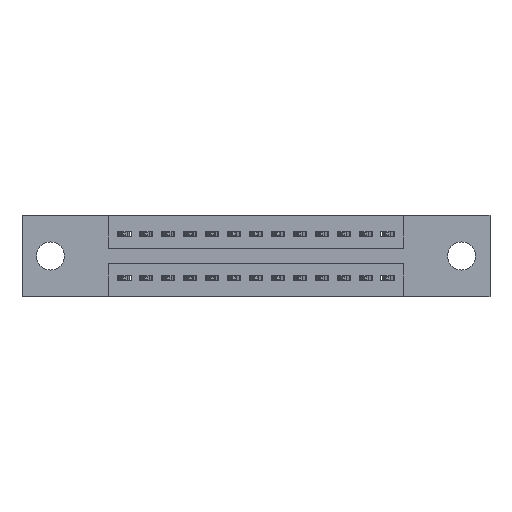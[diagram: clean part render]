
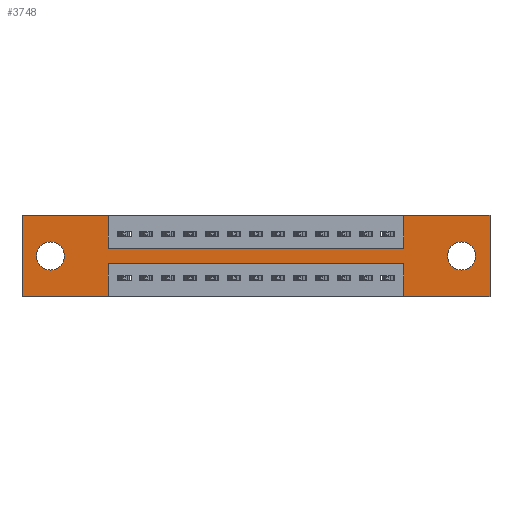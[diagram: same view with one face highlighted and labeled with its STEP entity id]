
A CAD part, front view. The second image highlights one B-rep face of the part: STEP entity #3748.
In plain terms, the highlighted planar face has unit normal (0, -1, 0).
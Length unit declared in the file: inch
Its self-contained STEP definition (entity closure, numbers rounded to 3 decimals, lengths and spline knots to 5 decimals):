
#61 = EDGE_CURVE ( 'NONE', #3490, #3423, #10278, .T. ) ;
#77 = VERTEX_POINT ( 'NONE', #11691 ) ;
#317 = DIRECTION ( 'NONE',  ( 0., 0., -1. ) ) ;
#356 = CARTESIAN_POINT ( 'NONE',  ( 0., 0., -0.37 ) ) ;
#383 = ORIENTED_EDGE ( 'NONE', *, *, #7710, .F. ) ;
#387 = VERTEX_POINT ( 'NONE', #8515 ) ;
#494 = DIRECTION ( 'NONE',  ( 0., 0., 1. ) ) ;
#524 = CARTESIAN_POINT ( 'NONE',  ( 0.13, 0., -0.185 ) ) ;
#543 = LINE ( 'NONE', #12159, #6457 ) ;
#552 = CARTESIAN_POINT ( 'NONE',  ( 1.7425, 0., 0. ) ) ;
#1044 = EDGE_CURVE ( 'NONE', #3004, #1251, #7736, .T. ) ;
#1169 = VERTEX_POINT ( 'NONE', #552 ) ;
#1219 = ORIENTED_EDGE ( 'NONE', *, *, #2390, .F. ) ;
#1251 = VERTEX_POINT ( 'NONE', #9426 ) ;
#1359 = DIRECTION ( 'NONE',  ( 1., 0., 0. ) ) ;
#1481 = CARTESIAN_POINT ( 'NONE',  ( 0., 0., 0. ) ) ;
#1528 = DIRECTION ( 'NONE',  ( 0., 0., 1. ) ) ;
#1544 = CIRCLE ( 'NONE', #6856, 0.064 ) ;
#1558 = DIRECTION ( 'NONE',  ( -1., 0., 0. ) ) ;
#1651 = EDGE_CURVE ( 'NONE', #13113, #387, #5462, .T. ) ;
#1752 = FACE_OUTER_BOUND ( 'NONE', #13735, .T. ) ;
#1858 = DIRECTION ( 'NONE',  ( 0., 0., 1. ) ) ;
#1883 = CARTESIAN_POINT ( 'NONE',  ( 2.135, 0., -0.37 ) ) ;
#1979 = VECTOR ( 'NONE', #1359, 39.37008 ) ;
#2236 = CARTESIAN_POINT ( 'NONE',  ( 2.135, 0., 0. ) ) ;
#2390 = EDGE_CURVE ( 'NONE', #8457, #4917, #5078, .T. ) ;
#2726 = CARTESIAN_POINT ( 'NONE',  ( 0.3925, 0., -0.15 ) ) ;
#2731 = CARTESIAN_POINT ( 'NONE',  ( 1.7425, 0., 0. ) ) ;
#2980 = LINE ( 'NONE', #12984, #13831 ) ;
#2991 = ORIENTED_EDGE ( 'NONE', *, *, #12994, .T. ) ;
#3004 = VERTEX_POINT ( 'NONE', #14059 ) ;
#3158 = AXIS2_PLACEMENT_3D ( 'NONE', #10783, #7246, #7576 ) ;
#3216 = CARTESIAN_POINT ( 'NONE',  ( 0.13, 0., -0.249 ) ) ;
#3333 = ORIENTED_EDGE ( 'NONE', *, *, #11763, .F. ) ;
#3414 = DIRECTION ( 'NONE',  ( 0., 0., -1. ) ) ;
#3423 = VERTEX_POINT ( 'NONE', #8905 ) ;
#3490 = VERTEX_POINT ( 'NONE', #7966 ) ;
#3528 = EDGE_CURVE ( 'NONE', #3423, #3490, #1544, .T. ) ;
#3617 = VECTOR ( 'NONE', #1558, 39.37008 ) ;
#3696 = ORIENTED_EDGE ( 'NONE', *, *, #7559, .F. ) ;
#3748 = ADVANCED_FACE ( 'NONE', ( #7465, #5228, #1752 ), #5443, .T. ) ;
#3947 = LINE ( 'NONE', #6393, #6555 ) ;
#4068 = ORIENTED_EDGE ( 'NONE', *, *, #10423, .F. ) ;
#4096 = VECTOR ( 'NONE', #12613, 39.37008 ) ;
#4218 = VECTOR ( 'NONE', #13090, 39.37008 ) ;
#4289 = EDGE_CURVE ( 'NONE', #1251, #9823, #12178, .T. ) ;
#4331 = AXIS2_PLACEMENT_3D ( 'NONE', #5634, #5425, #5401 ) ;
#4567 = LINE ( 'NONE', #12171, #4218 ) ;
#4735 = CARTESIAN_POINT ( 'NONE',  ( 0.3925, 0., -0.22 ) ) ;
#4736 = DIRECTION ( 'NONE',  ( 0., 0., 1. ) ) ;
#4754 = DIRECTION ( 'NONE',  ( 0., 1., 0. ) ) ;
#4758 = CARTESIAN_POINT ( 'NONE',  ( 0.13, 0., -0.185 ) ) ;
#4917 = VERTEX_POINT ( 'NONE', #12175 ) ;
#5078 = LINE ( 'NONE', #1481, #1979 ) ;
#5228 = FACE_BOUND ( 'NONE', #8115, .T. ) ;
#5284 = CARTESIAN_POINT ( 'NONE',  ( 0., 0., 0. ) ) ;
#5348 = EDGE_CURVE ( 'NONE', #4917, #5632, #13626, .T. ) ;
#5401 = DIRECTION ( 'NONE',  ( 0., 0., -1. ) ) ;
#5425 = DIRECTION ( 'NONE',  ( 0., -1., 0. ) ) ;
#5443 = PLANE ( 'NONE',  #4331 ) ;
#5462 = CIRCLE ( 'NONE', #7497, 0.064 ) ;
#5632 = VERTEX_POINT ( 'NONE', #2726 ) ;
#5634 = CARTESIAN_POINT ( 'NONE',  ( 0., 0., -0.37 ) ) ;
#5644 = ORIENTED_EDGE ( 'NONE', *, *, #3528, .T. ) ;
#5851 = LINE ( 'NONE', #2731, #11211 ) ;
#5983 = ORIENTED_EDGE ( 'NONE', *, *, #1651, .T. ) ;
#6333 = ORIENTED_EDGE ( 'NONE', *, *, #11100, .F. ) ;
#6393 = CARTESIAN_POINT ( 'NONE',  ( 0., 0., 0. ) ) ;
#6457 = VECTOR ( 'NONE', #13072, 39.37008 ) ;
#6555 = VECTOR ( 'NONE', #494, 39.37008 ) ;
#6856 = AXIS2_PLACEMENT_3D ( 'NONE', #7679, #7663, #7643 ) ;
#6888 = CARTESIAN_POINT ( 'NONE',  ( 0.3925, 0., -0.37 ) ) ;
#6919 = DIRECTION ( 'NONE',  ( -1., 0., 0. ) ) ;
#6994 = EDGE_CURVE ( 'NONE', #9823, #8457, #3947, .T. ) ;
#7037 = VERTEX_POINT ( 'NONE', #1883 ) ;
#7058 = CARTESIAN_POINT ( 'NONE',  ( 2.135, 0., 0. ) ) ;
#7246 = DIRECTION ( 'NONE',  ( 0., 1., 0. ) ) ;
#7379 = VECTOR ( 'NONE', #317, 39.37008 ) ;
#7380 = ORIENTED_EDGE ( 'NONE', *, *, #6994, .F. ) ;
#7465 = FACE_BOUND ( 'NONE', #13155, .T. ) ;
#7497 = AXIS2_PLACEMENT_3D ( 'NONE', #4758, #4754, #4736 ) ;
#7559 = EDGE_CURVE ( 'NONE', #8117, #1169, #5851, .T. ) ;
#7576 = DIRECTION ( 'NONE',  ( 0., 0., -1. ) ) ;
#7643 = DIRECTION ( 'NONE',  ( 0., 0., -1. ) ) ;
#7663 = DIRECTION ( 'NONE',  ( 0., 1., 0. ) ) ;
#7679 = CARTESIAN_POINT ( 'NONE',  ( 2.005, 0., -0.185 ) ) ;
#7685 = LINE ( 'NONE', #2236, #12773 ) ;
#7710 = EDGE_CURVE ( 'NONE', #1169, #11822, #7771, .T. ) ;
#7736 = LINE ( 'NONE', #6888, #7379 ) ;
#7771 = LINE ( 'NONE', #5284, #4096 ) ;
#7966 = CARTESIAN_POINT ( 'NONE',  ( 2.005, 0., -0.249 ) ) ;
#8115 = EDGE_LOOP ( 'NONE', ( #2991, #5983 ) ) ;
#8117 = VERTEX_POINT ( 'NONE', #9492 ) ;
#8205 = CIRCLE ( 'NONE', #9465, 0.064 ) ;
#8457 = VERTEX_POINT ( 'NONE', #11938 ) ;
#8515 = CARTESIAN_POINT ( 'NONE',  ( 0.13, 0., -0.121 ) ) ;
#8614 = ORIENTED_EDGE ( 'NONE', *, *, #61, .T. ) ;
#8682 = DIRECTION ( 'NONE',  ( 0., 1., 0. ) ) ;
#8905 = CARTESIAN_POINT ( 'NONE',  ( 2.005, 0., -0.121 ) ) ;
#8969 = ORIENTED_EDGE ( 'NONE', *, *, #1044, .F. ) ;
#9307 = ORIENTED_EDGE ( 'NONE', *, *, #9521, .F. ) ;
#9426 = CARTESIAN_POINT ( 'NONE',  ( 0.3925, 0., -0.37 ) ) ;
#9465 = AXIS2_PLACEMENT_3D ( 'NONE', #524, #8682, #1858 ) ;
#9492 = CARTESIAN_POINT ( 'NONE',  ( 1.7425, 0., -0.15 ) ) ;
#9521 = EDGE_CURVE ( 'NONE', #7037, #77, #4567, .T. ) ;
#9823 = VERTEX_POINT ( 'NONE', #356 ) ;
#9856 = VERTEX_POINT ( 'NONE', #12573 ) ;
#10163 = DIRECTION ( 'NONE',  ( 0., 0., 1. ) ) ;
#10240 = ORIENTED_EDGE ( 'NONE', *, *, #4289, .F. ) ;
#10271 = DIRECTION ( 'NONE',  ( 0., 0., -1. ) ) ;
#10278 = CIRCLE ( 'NONE', #3158, 0.064 ) ;
#10312 = CARTESIAN_POINT ( 'NONE',  ( 0.3925, 0., 0. ) ) ;
#10423 = EDGE_CURVE ( 'NONE', #5632, #8117, #543, .T. ) ;
#10783 = CARTESIAN_POINT ( 'NONE',  ( 2.005, 0., -0.185 ) ) ;
#11023 = LINE ( 'NONE', #4735, #13235 ) ;
#11100 = EDGE_CURVE ( 'NONE', #77, #9856, #2980, .T. ) ;
#11110 = VECTOR ( 'NONE', #10271, 39.37008 ) ;
#11211 = VECTOR ( 'NONE', #1528, 39.37008 ) ;
#11691 = CARTESIAN_POINT ( 'NONE',  ( 1.7425, 0., -0.37 ) ) ;
#11763 = EDGE_CURVE ( 'NONE', #9856, #3004, #11023, .T. ) ;
#11822 = VERTEX_POINT ( 'NONE', #7058 ) ;
#11938 = CARTESIAN_POINT ( 'NONE',  ( 0., 0., 0. ) ) ;
#11939 = ORIENTED_EDGE ( 'NONE', *, *, #12770, .F. ) ;
#12159 = CARTESIAN_POINT ( 'NONE',  ( 0.3925, 0., -0.15 ) ) ;
#12171 = CARTESIAN_POINT ( 'NONE',  ( 0., 0., -0.37 ) ) ;
#12175 = CARTESIAN_POINT ( 'NONE',  ( 0.3925, 0., 0. ) ) ;
#12178 = LINE ( 'NONE', #12349, #3617 ) ;
#12349 = CARTESIAN_POINT ( 'NONE',  ( 0., 0., -0.37 ) ) ;
#12532 = ORIENTED_EDGE ( 'NONE', *, *, #5348, .F. ) ;
#12573 = CARTESIAN_POINT ( 'NONE',  ( 1.7425, 0., -0.22 ) ) ;
#12613 = DIRECTION ( 'NONE',  ( 1., 0., 0. ) ) ;
#12770 = EDGE_CURVE ( 'NONE', #11822, #7037, #7685, .T. ) ;
#12773 = VECTOR ( 'NONE', #3414, 39.37008 ) ;
#12984 = CARTESIAN_POINT ( 'NONE',  ( 1.7425, 0., -0.37 ) ) ;
#12994 = EDGE_CURVE ( 'NONE', #387, #13113, #8205, .T. ) ;
#13072 = DIRECTION ( 'NONE',  ( 1., 0., 0. ) ) ;
#13090 = DIRECTION ( 'NONE',  ( -1., 0., 0. ) ) ;
#13113 = VERTEX_POINT ( 'NONE', #3216 ) ;
#13155 = EDGE_LOOP ( 'NONE', ( #5644, #8614 ) ) ;
#13235 = VECTOR ( 'NONE', #6919, 39.37008 ) ;
#13626 = LINE ( 'NONE', #10312, #11110 ) ;
#13735 = EDGE_LOOP ( 'NONE', ( #8969, #3333, #6333, #9307, #11939, #383, #3696, #4068, #12532, #1219, #7380, #10240 ) ) ;
#13831 = VECTOR ( 'NONE', #10163, 39.37008 ) ;
#14059 = CARTESIAN_POINT ( 'NONE',  ( 0.3925, 0., -0.22 ) ) ;
